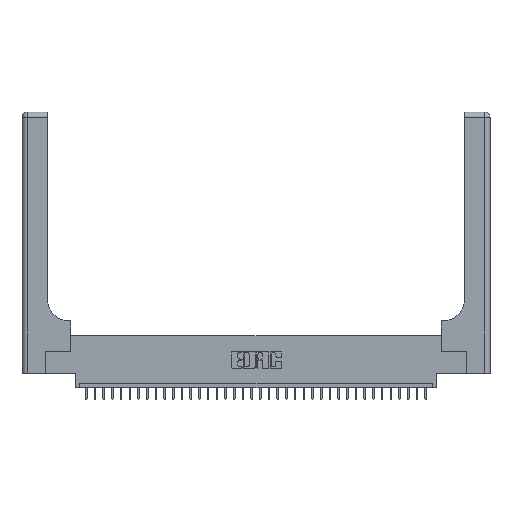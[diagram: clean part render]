
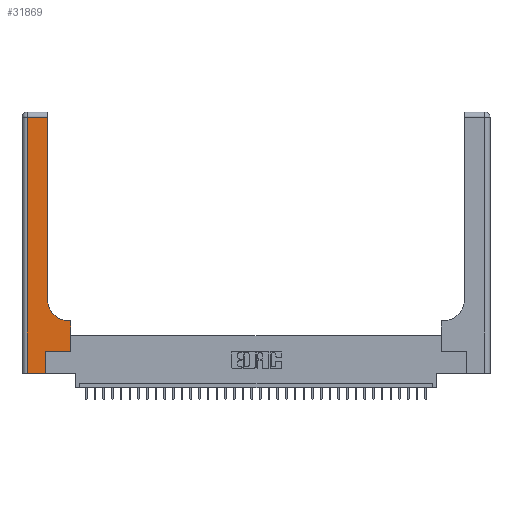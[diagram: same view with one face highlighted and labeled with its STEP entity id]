
A CAD part, top view. The second image highlights one B-rep face of the part: STEP entity #31869.
In plain terms, the highlighted planar face has unit normal (0, 0, 1).
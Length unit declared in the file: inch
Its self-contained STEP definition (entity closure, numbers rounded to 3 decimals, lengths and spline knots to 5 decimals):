
#72 = DIRECTION ( 'NONE',  ( -1., 0., 0. ) ) ;
#1788 = VERTEX_POINT ( 'NONE', #29829 ) ;
#1847 = ORIENTED_EDGE ( 'NONE', *, *, #18626, .T. ) ;
#1853 = VECTOR ( 'NONE', #5157, 39.37008 ) ;
#2089 = CARTESIAN_POINT ( 'NONE',  ( 0.2915, 0.85, 0.37 ) ) ;
#2372 = DIRECTION ( 'NONE',  ( -1., 0., 0. ) ) ;
#2575 = CARTESIAN_POINT ( 'NONE',  ( 0.269, 0., 0.37 ) ) ;
#2783 = DIRECTION ( 'NONE',  ( 0., 1., 0. ) ) ;
#2787 = PLANE ( 'NONE',  #7186 ) ;
#3134 = LINE ( 'NONE', #16535, #13175 ) ;
#3154 = VERTEX_POINT ( 'NONE', #12619 ) ;
#3368 = VERTEX_POINT ( 'NONE', #25198 ) ;
#3377 = CARTESIAN_POINT ( 'NONE',  ( 0.06, 3., 0.37 ) ) ;
#3409 = VERTEX_POINT ( 'NONE', #22860 ) ;
#3454 = VERTEX_POINT ( 'NONE', #6231 ) ;
#4879 = CARTESIAN_POINT ( 'NONE',  ( 0., 2.94, 0.37 ) ) ;
#5157 = DIRECTION ( 'NONE',  ( 1., 0., 0. ) ) ;
#5423 = VECTOR ( 'NONE', #11610, 39.37008 ) ;
#6231 = CARTESIAN_POINT ( 'NONE',  ( 0.06, 2.94, 0.37 ) ) ;
#7186 = AXIS2_PLACEMENT_3D ( 'NONE', #24827, #22129, #72 ) ;
#7304 = CARTESIAN_POINT ( 'NONE',  ( 0.5415, 0.85, 0.37 ) ) ;
#7426 = LINE ( 'NONE', #4879, #14567 ) ;
#7535 = CARTESIAN_POINT ( 'NONE',  ( 0., 0., 0.37 ) ) ;
#8325 = CARTESIAN_POINT ( 'NONE',  ( 0.269, 0.25, 0.37 ) ) ;
#8329 = VECTOR ( 'NONE', #2372, 39.37008 ) ;
#10094 = VECTOR ( 'NONE', #14409, 39.37008 ) ;
#10382 = ORIENTED_EDGE ( 'NONE', *, *, #16475, .T. ) ;
#10483 = DIRECTION ( 'NONE',  ( -1., 0., 0. ) ) ;
#10559 = ORIENTED_EDGE ( 'NONE', *, *, #15791, .T. ) ;
#11439 = FACE_OUTER_BOUND ( 'NONE', #18053, .T. ) ;
#11610 = DIRECTION ( 'NONE',  ( 0., 1., 0. ) ) ;
#12451 = VECTOR ( 'NONE', #2783, 39.37008 ) ;
#12619 = CARTESIAN_POINT ( 'NONE',  ( 0.5585, 0.25, 0.37 ) ) ;
#13175 = VECTOR ( 'NONE', #22130, 39.37008 ) ;
#13237 = EDGE_CURVE ( 'NONE', #3368, #3454, #7426, .T. ) ;
#13538 = ORIENTED_EDGE ( 'NONE', *, *, #21652, .T. ) ;
#13923 = LINE ( 'NONE', #33105, #8329 ) ;
#13940 = DIRECTION ( 'NONE',  ( 1., 0., 0. ) ) ;
#13991 = EDGE_CURVE ( 'NONE', #1788, #18515, #27309, .T. ) ;
#14409 = DIRECTION ( 'NONE',  ( 0., -1., 0. ) ) ;
#14419 = ORIENTED_EDGE ( 'NONE', *, *, #13237, .T. ) ;
#14567 = VECTOR ( 'NONE', #10483, 39.37008 ) ;
#15081 = DIRECTION ( 'NONE',  ( 0., 0., -1. ) ) ;
#15536 = VERTEX_POINT ( 'NONE', #24666 ) ;
#15791 = EDGE_CURVE ( 'NONE', #3409, #1788, #13923, .T. ) ;
#16475 = EDGE_CURVE ( 'NONE', #3454, #15536, #30521, .T. ) ;
#16527 = LINE ( 'NONE', #27539, #12451 ) ;
#16535 = CARTESIAN_POINT ( 'NONE',  ( 0.269, 0., 0.37 ) ) ;
#17489 = EDGE_CURVE ( 'NONE', #18515, #3368, #19412, .T. ) ;
#17952 = EDGE_CURVE ( 'NONE', #19367, #3154, #33123, .T. ) ;
#18053 = EDGE_LOOP ( 'NONE', ( #21757, #14419, #10382, #18864, #13538, #26986, #1847, #10559, #34872 ) ) ;
#18515 = VERTEX_POINT ( 'NONE', #2089 ) ;
#18626 = EDGE_CURVE ( 'NONE', #3154, #3409, #16527, .T. ) ;
#18864 = ORIENTED_EDGE ( 'NONE', *, *, #28791, .T. ) ;
#19367 = VERTEX_POINT ( 'NONE', #35637 ) ;
#19412 = LINE ( 'NONE', #30270, #5423 ) ;
#21652 = EDGE_CURVE ( 'NONE', #21990, #19367, #3134, .T. ) ;
#21757 = ORIENTED_EDGE ( 'NONE', *, *, #17489, .T. ) ;
#21990 = VERTEX_POINT ( 'NONE', #2575 ) ;
#22129 = DIRECTION ( 'NONE',  ( 0., 0., -1. ) ) ;
#22130 = DIRECTION ( 'NONE',  ( 0., 1., 0. ) ) ;
#22860 = CARTESIAN_POINT ( 'NONE',  ( 0.5585, 0.6, 0.37 ) ) ;
#24666 = CARTESIAN_POINT ( 'NONE',  ( 0.06, 0., 0.37 ) ) ;
#24827 = CARTESIAN_POINT ( 'NONE',  ( 0., 3., 0.37 ) ) ;
#25198 = CARTESIAN_POINT ( 'NONE',  ( 0.2915, 2.94, 0.37 ) ) ;
#26637 = DIRECTION ( 'NONE',  ( 1., 0., 0. ) ) ;
#26986 = ORIENTED_EDGE ( 'NONE', *, *, #17952, .T. ) ;
#27309 = CIRCLE ( 'NONE', #28474, 0.25 ) ;
#27539 = CARTESIAN_POINT ( 'NONE',  ( 0.5585, 0.25, 0.37 ) ) ;
#28474 = AXIS2_PLACEMENT_3D ( 'NONE', #7304, #15081, #26637 ) ;
#28791 = EDGE_CURVE ( 'NONE', #15536, #21990, #35055, .T. ) ;
#29750 = VECTOR ( 'NONE', #13940, 39.37008 ) ;
#29829 = CARTESIAN_POINT ( 'NONE',  ( 0.5415, 0.6, 0.37 ) ) ;
#30270 = CARTESIAN_POINT ( 'NONE',  ( 0.2915, 3., 0.37 ) ) ;
#30521 = LINE ( 'NONE', #3377, #10094 ) ;
#31869 = ADVANCED_FACE ( 'NONE', ( #11439 ), #2787, .F. ) ;
#33105 = CARTESIAN_POINT ( 'NONE',  ( 0.2915, 0.6, 0.37 ) ) ;
#33123 = LINE ( 'NONE', #8325, #29750 ) ;
#34872 = ORIENTED_EDGE ( 'NONE', *, *, #13991, .T. ) ;
#35055 = LINE ( 'NONE', #7535, #1853 ) ;
#35637 = CARTESIAN_POINT ( 'NONE',  ( 0.269, 0.25, 0.37 ) ) ;
